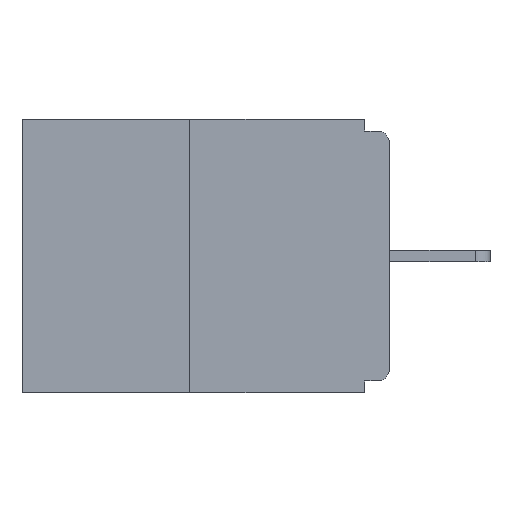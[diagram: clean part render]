
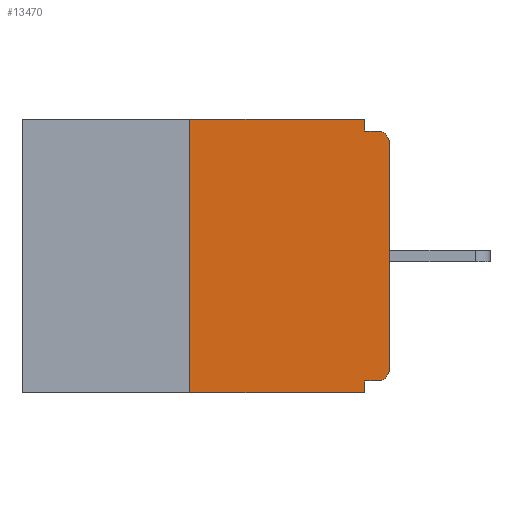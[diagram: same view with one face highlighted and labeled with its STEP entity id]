
A CAD part, left-side view. The second image highlights one B-rep face of the part: STEP entity #13470.
In plain terms, the highlighted planar face has unit normal (-1, 0, 0).
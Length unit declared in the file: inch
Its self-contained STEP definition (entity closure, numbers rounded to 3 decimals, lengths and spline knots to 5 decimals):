
#205 = EDGE_CURVE ( 'NONE', #12711, #11289, #365, .T. ) ;
#266 = CARTESIAN_POINT ( 'NONE',  ( 0., 0.015, -0.015 ) ) ;
#316 = LINE ( 'NONE', #4556, #6347 ) ;
#365 = LINE ( 'NONE', #4245, #3248 ) ;
#734 = DIRECTION ( 'NONE',  ( 0., -1., 0. ) ) ;
#821 = EDGE_CURVE ( 'NONE', #4341, #13429, #919, .T. ) ;
#919 = LINE ( 'NONE', #1825, #12776 ) ;
#1231 = CARTESIAN_POINT ( 'NONE',  ( 0., 0.031, -0.015 ) ) ;
#1293 = ORIENTED_EDGE ( 'NONE', *, *, #4533, .F. ) ;
#1530 = DIRECTION ( 'NONE',  ( 0., -1., 0. ) ) ;
#1821 = DIRECTION ( 'NONE',  ( 0., 0., -1. ) ) ;
#1825 = CARTESIAN_POINT ( 'NONE',  ( 0., 0.46, -0.343 ) ) ;
#2207 = VECTOR ( 'NONE', #11324, 39.37008 ) ;
#2286 = ORIENTED_EDGE ( 'NONE', *, *, #205, .F. ) ;
#2453 = VECTOR ( 'NONE', #1530, 39.37008 ) ;
#2455 = ORIENTED_EDGE ( 'NONE', *, *, #2464, .F. ) ;
#2464 = EDGE_CURVE ( 'NONE', #4341, #12891, #316, .T. ) ;
#2468 = ORIENTED_EDGE ( 'NONE', *, *, #7709, .T. ) ;
#2617 = VERTEX_POINT ( 'NONE', #13712 ) ;
#2775 = DIRECTION ( 'NONE',  ( 0., 0., -1. ) ) ;
#3248 = VECTOR ( 'NONE', #4275, 39.37008 ) ;
#3470 = VECTOR ( 'NONE', #8805, 39.37008 ) ;
#3536 = DIRECTION ( 'NONE',  ( 0., 0., 1. ) ) ;
#3612 = CARTESIAN_POINT ( 'NONE',  ( 0., 0.031, -0.328 ) ) ;
#3654 = VERTEX_POINT ( 'NONE', #266 ) ;
#3856 = LINE ( 'NONE', #11665, #3470 ) ;
#4245 = CARTESIAN_POINT ( 'NONE',  ( 0., 0., -0.328 ) ) ;
#4275 = DIRECTION ( 'NONE',  ( 0., 1., 0. ) ) ;
#4341 = VERTEX_POINT ( 'NONE', #9806 ) ;
#4533 = EDGE_CURVE ( 'NONE', #12891, #2617, #13483, .T. ) ;
#4556 = CARTESIAN_POINT ( 'NONE',  ( 0., 0.25, 0. ) ) ;
#4809 = CIRCLE ( 'NONE', #14400, 0.015 ) ;
#4917 = DIRECTION ( 'NONE',  ( -1., 0., 0. ) ) ;
#5192 = CARTESIAN_POINT ( 'NONE',  ( 0., 0.031, -0.343 ) ) ;
#5346 = VERTEX_POINT ( 'NONE', #12089 ) ;
#5403 = CARTESIAN_POINT ( 'NONE',  ( 0., 0.46, 0. ) ) ;
#5690 = CIRCLE ( 'NONE', #9532, 0.015 ) ;
#5879 = EDGE_CURVE ( 'NONE', #14227, #5346, #3856, .T. ) ;
#6347 = VECTOR ( 'NONE', #3536, 39.37008 ) ;
#6759 = DIRECTION ( 'NONE',  ( 0., 0., -1. ) ) ;
#6768 = CARTESIAN_POINT ( 'NONE',  ( 0., 0.25, 0. ) ) ;
#6799 = DIRECTION ( 'NONE',  ( -1., 0., 0. ) ) ;
#6812 = CARTESIAN_POINT ( 'NONE',  ( 0., 0.015, -0.03 ) ) ;
#7084 = ORIENTED_EDGE ( 'NONE', *, *, #11221, .F. ) ;
#7482 = EDGE_LOOP ( 'NONE', ( #1293, #2455, #9804, #7084, #2286, #8547, #12481, #2468, #14190, #9472 ) ) ;
#7660 = PLANE ( 'NONE',  #9112 ) ;
#7709 = EDGE_CURVE ( 'NONE', #5346, #3654, #4809, .T. ) ;
#7716 = VECTOR ( 'NONE', #2775, 39.37008 ) ;
#8547 = ORIENTED_EDGE ( 'NONE', *, *, #10024, .T. ) ;
#8763 = CARTESIAN_POINT ( 'NONE',  ( 0., 0.015, -0.328 ) ) ;
#8805 = DIRECTION ( 'NONE',  ( 0., 0., 1. ) ) ;
#8889 = DIRECTION ( 'NONE',  ( 1., 0., 0. ) ) ;
#9112 = AXIS2_PLACEMENT_3D ( 'NONE', #5403, #8889, #1821 ) ;
#9113 = CARTESIAN_POINT ( 'NONE',  ( 0., 0., -0.313 ) ) ;
#9472 = ORIENTED_EDGE ( 'NONE', *, *, #14014, .F. ) ;
#9532 = AXIS2_PLACEMENT_3D ( 'NONE', #11724, #4917, #12739 ) ;
#9804 = ORIENTED_EDGE ( 'NONE', *, *, #821, .T. ) ;
#9806 = CARTESIAN_POINT ( 'NONE',  ( 0., 0.25, -0.343 ) ) ;
#10024 = EDGE_CURVE ( 'NONE', #12711, #14227, #5690, .T. ) ;
#10614 = FACE_OUTER_BOUND ( 'NONE', #7482, .T. ) ;
#10706 = VERTEX_POINT ( 'NONE', #1231 ) ;
#10762 = LINE ( 'NONE', #5192, #7716 ) ;
#10981 = DIRECTION ( 'NONE',  ( 0., 0., -1. ) ) ;
#11221 = EDGE_CURVE ( 'NONE', #11289, #13429, #10762, .T. ) ;
#11289 = VERTEX_POINT ( 'NONE', #3612 ) ;
#11324 = DIRECTION ( 'NONE',  ( 0., -1., 0. ) ) ;
#11336 = CARTESIAN_POINT ( 'NONE',  ( 0., 0.46, 0. ) ) ;
#11497 = EDGE_CURVE ( 'NONE', #10706, #3654, #14329, .T. ) ;
#11665 = CARTESIAN_POINT ( 'NONE',  ( 0., 0., 0. ) ) ;
#11724 = CARTESIAN_POINT ( 'NONE',  ( 0., 0.015, -0.313 ) ) ;
#12089 = CARTESIAN_POINT ( 'NONE',  ( 0., 0., -0.03 ) ) ;
#12481 = ORIENTED_EDGE ( 'NONE', *, *, #5879, .T. ) ;
#12711 = VERTEX_POINT ( 'NONE', #8763 ) ;
#12739 = DIRECTION ( 'NONE',  ( 0., 0., -1. ) ) ;
#12776 = VECTOR ( 'NONE', #734, 39.37008 ) ;
#12891 = VERTEX_POINT ( 'NONE', #6768 ) ;
#13024 = VECTOR ( 'NONE', #10981, 39.37008 ) ;
#13053 = CARTESIAN_POINT ( 'NONE',  ( 0., 0.031, -0.343 ) ) ;
#13333 = LINE ( 'NONE', #13998, #13024 ) ;
#13429 = VERTEX_POINT ( 'NONE', #13053 ) ;
#13470 = ADVANCED_FACE ( 'NONE', ( #10614 ), #7660, .F. ) ;
#13483 = LINE ( 'NONE', #11336, #2207 ) ;
#13712 = CARTESIAN_POINT ( 'NONE',  ( 0., 0.031, 0. ) ) ;
#13876 = CARTESIAN_POINT ( 'NONE',  ( 0., 0., -0.015 ) ) ;
#13998 = CARTESIAN_POINT ( 'NONE',  ( 0., 0.031, 0. ) ) ;
#14014 = EDGE_CURVE ( 'NONE', #2617, #10706, #13333, .T. ) ;
#14190 = ORIENTED_EDGE ( 'NONE', *, *, #11497, .F. ) ;
#14227 = VERTEX_POINT ( 'NONE', #9113 ) ;
#14329 = LINE ( 'NONE', #13876, #2453 ) ;
#14400 = AXIS2_PLACEMENT_3D ( 'NONE', #6812, #6799, #6759 ) ;
